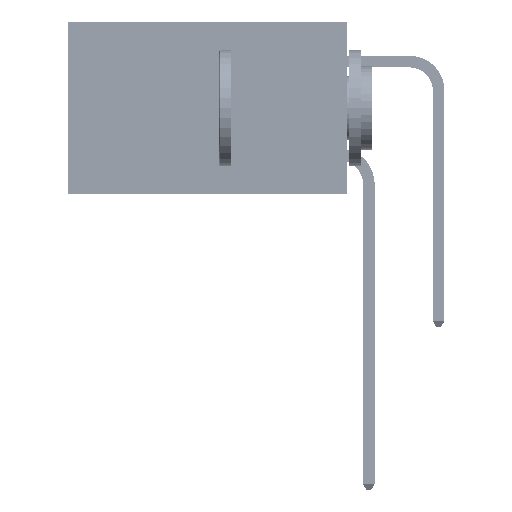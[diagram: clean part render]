
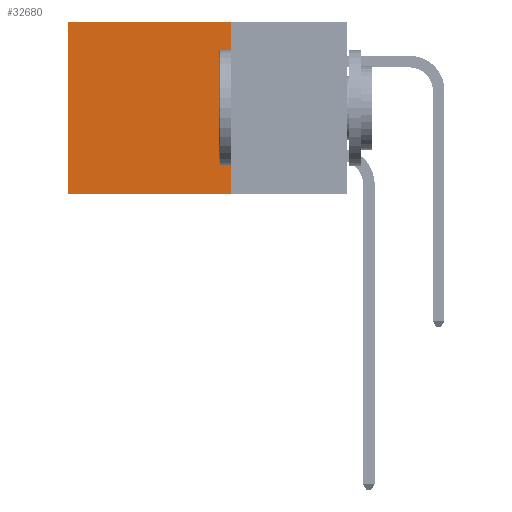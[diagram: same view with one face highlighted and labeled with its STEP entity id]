
A CAD part, left-side view. The second image highlights one B-rep face of the part: STEP entity #32680.
In plain terms, the highlighted planar face has unit normal (-1, 0, 0).
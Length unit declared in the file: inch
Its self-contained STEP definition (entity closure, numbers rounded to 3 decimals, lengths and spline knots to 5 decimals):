
#1084 = VECTOR ( 'NONE', #27555, 39.37008 ) ;
#1389 = EDGE_CURVE ( 'NONE', #40180, #36508, #40909, .T. ) ;
#2164 = LINE ( 'NONE', #46247, #33946 ) ;
#2799 = VERTEX_POINT ( 'NONE', #41933 ) ;
#6012 = ORIENTED_EDGE ( 'NONE', *, *, #1389, .T. ) ;
#6067 = DIRECTION ( 'NONE',  ( 0., 0., -1. ) ) ;
#6339 = DIRECTION ( 'NONE',  ( 0., 1., 0. ) ) ;
#9424 = FACE_OUTER_BOUND ( 'NONE', #29940, .T. ) ;
#10560 = EDGE_CURVE ( 'NONE', #2799, #36508, #2164, .T. ) ;
#11402 = DIRECTION ( 'NONE',  ( 0., 0., -1. ) ) ;
#11564 = CARTESIAN_POINT ( 'NONE',  ( 0.2875, 0.25, 0. ) ) ;
#13006 = LINE ( 'NONE', #21957, #1084 ) ;
#16096 = DIRECTION ( 'NONE',  ( 0., 0., -1. ) ) ;
#20280 = EDGE_CURVE ( 'NONE', #29635, #2799, #36092, .T. ) ;
#21957 = CARTESIAN_POINT ( 'NONE',  ( 0.2875, 0.25, 0. ) ) ;
#25890 = DIRECTION ( 'NONE',  ( 1., 0., 0. ) ) ;
#27555 = DIRECTION ( 'NONE',  ( 0., 1., 0. ) ) ;
#29224 = AXIS2_PLACEMENT_3D ( 'NONE', #29709, #25890, #6067 ) ;
#29635 = VERTEX_POINT ( 'NONE', #35261 ) ;
#29709 = CARTESIAN_POINT ( 'NONE',  ( 0.2875, 0.25, 0. ) ) ;
#29940 = EDGE_LOOP ( 'NONE', ( #6012, #30616, #45803, #42081 ) ) ;
#30616 = ORIENTED_EDGE ( 'NONE', *, *, #10560, .F. ) ;
#30903 = CARTESIAN_POINT ( 'NONE',  ( 0.2875, 0.6, 0. ) ) ;
#32680 = ADVANCED_FACE ( 'NONE', ( #9424 ), #33542, .F. ) ;
#33542 = PLANE ( 'NONE',  #29224 ) ;
#33946 = VECTOR ( 'NONE', #6339, 39.37008 ) ;
#35211 = EDGE_CURVE ( 'NONE', #29635, #40180, #13006, .T. ) ;
#35261 = CARTESIAN_POINT ( 'NONE',  ( 0.2875, 0.25, 0. ) ) ;
#36092 = LINE ( 'NONE', #11564, #46636 ) ;
#36508 = VERTEX_POINT ( 'NONE', #42527 ) ;
#37178 = VECTOR ( 'NONE', #16096, 39.37008 ) ;
#39706 = CARTESIAN_POINT ( 'NONE',  ( 0.2875, 0.6, 0. ) ) ;
#40180 = VERTEX_POINT ( 'NONE', #30903 ) ;
#40909 = LINE ( 'NONE', #39706, #37178 ) ;
#41933 = CARTESIAN_POINT ( 'NONE',  ( 0.2875, 0.25, -0.37 ) ) ;
#42081 = ORIENTED_EDGE ( 'NONE', *, *, #35211, .T. ) ;
#42527 = CARTESIAN_POINT ( 'NONE',  ( 0.2875, 0.6, -0.37 ) ) ;
#45803 = ORIENTED_EDGE ( 'NONE', *, *, #20280, .F. ) ;
#46247 = CARTESIAN_POINT ( 'NONE',  ( 0.2875, 0.25, -0.37 ) ) ;
#46636 = VECTOR ( 'NONE', #11402, 39.37008 ) ;
